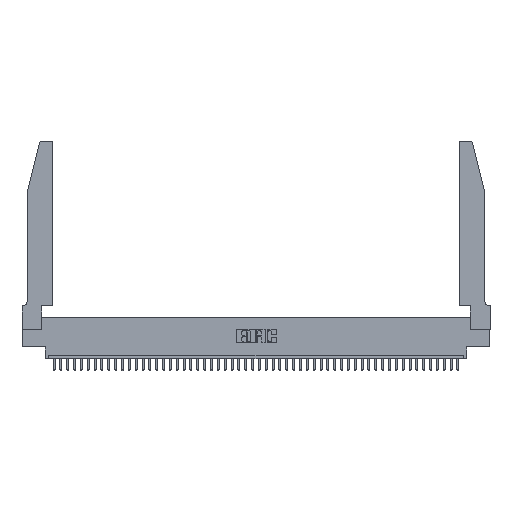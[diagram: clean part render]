
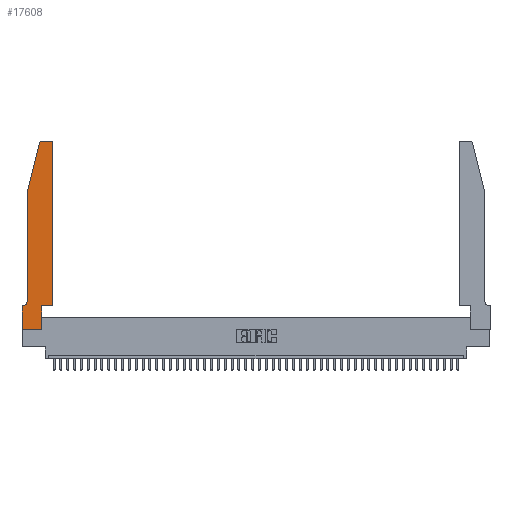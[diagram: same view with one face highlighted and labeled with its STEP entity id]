
A CAD part, top view. The second image highlights one B-rep face of the part: STEP entity #17608.
In plain terms, the highlighted planar face has unit normal (0, 0, 1).
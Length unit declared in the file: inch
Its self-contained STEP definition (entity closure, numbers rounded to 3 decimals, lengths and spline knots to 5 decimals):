
#796 = DIRECTION ( 'NONE',  ( -1., 0., 0. ) ) ;
#1854 = EDGE_CURVE ( 'NONE', #3958, #19040, #8267, .T. ) ;
#1920 = VECTOR ( 'NONE', #33301, 39.37008 ) ;
#2193 = ORIENTED_EDGE ( 'NONE', *, *, #1854, .T. ) ;
#2580 = AXIS2_PLACEMENT_3D ( 'NONE', #46384, #35325, #5504 ) ;
#2740 = DIRECTION ( 'NONE',  ( 0., 0., 1. ) ) ;
#3282 = AXIS2_PLACEMENT_3D ( 'NONE', #24497, #2740, #17591 ) ;
#3696 = CARTESIAN_POINT ( 'NONE',  ( 0.4505, 2.72, 0.37 ) ) ;
#3958 = VERTEX_POINT ( 'NONE', #18969 ) ;
#4555 = CARTESIAN_POINT ( 'NONE',  ( 0.0755, 2., 0.37 ) ) ;
#5211 = DIRECTION ( 'NONE',  ( 1., 0., 0. ) ) ;
#5504 = DIRECTION ( 'NONE',  ( 1., 0., 0. ) ) ;
#5720 = EDGE_CURVE ( 'NONE', #38643, #15057, #46241, .T. ) ;
#5841 = CARTESIAN_POINT ( 'NONE',  ( 0.2865, 0., 0.37 ) ) ;
#7037 = AXIS2_PLACEMENT_3D ( 'NONE', #32216, #13870, #47004 ) ;
#7317 = VECTOR ( 'NONE', #17837, 39.37008 ) ;
#7429 = DIRECTION ( 'NONE',  ( 0., 1., 0. ) ) ;
#8213 = ORIENTED_EDGE ( 'NONE', *, *, #44456, .T. ) ;
#8267 = LINE ( 'NONE', #10928, #1920 ) ;
#8400 = LINE ( 'NONE', #16300, #43541 ) ;
#8529 = EDGE_LOOP ( 'NONE', ( #19194, #29245, #8213, #34890, #30174, #2193, #38964, #18700, #45059, #26383, #11440, #38813 ) ) ;
#8995 = EDGE_CURVE ( 'NONE', #22311, #42083, #8400, .T. ) ;
#9408 = CARTESIAN_POINT ( 'NONE',  ( 0.0755, 2., 0.37 ) ) ;
#9685 = VERTEX_POINT ( 'NONE', #5841 ) ;
#10928 = CARTESIAN_POINT ( 'NONE',  ( 0.0755, 0.35, 0.37 ) ) ;
#11302 = DIRECTION ( 'NONE',  ( -0.239, -0.971, 0. ) ) ;
#11440 = ORIENTED_EDGE ( 'NONE', *, *, #37654, .T. ) ;
#12511 = LINE ( 'NONE', #28490, #7317 ) ;
#12840 = VECTOR ( 'NONE', #42834, 39.37008 ) ;
#13010 = VERTEX_POINT ( 'NONE', #25895 ) ;
#13510 = DIRECTION ( 'NONE',  ( 1., 0., 0. ) ) ;
#13753 = EDGE_CURVE ( 'NONE', #42083, #31272, #33928, .T. ) ;
#13870 = DIRECTION ( 'NONE',  ( 0., 0., -1. ) ) ;
#13898 = VECTOR ( 'NONE', #28652, 39.37008 ) ;
#15057 = VERTEX_POINT ( 'NONE', #15859 ) ;
#15088 = DIRECTION ( 'NONE',  ( 1., 0., 0. ) ) ;
#15477 = LINE ( 'NONE', #24240, #20648 ) ;
#15517 = EDGE_CURVE ( 'NONE', #29585, #20359, #20282, .T. ) ;
#15859 = CARTESIAN_POINT ( 'NONE',  ( 0.4505, 0.35, 0.37 ) ) ;
#16300 = CARTESIAN_POINT ( 'NONE',  ( 0.2605, 2.75, 0.37 ) ) ;
#16350 = LINE ( 'NONE', #43923, #18137 ) ;
#17591 = DIRECTION ( 'NONE',  ( 1., 0., 0. ) ) ;
#17608 = ADVANCED_FACE ( 'NONE', ( #18392 ), #24908, .T. ) ;
#17837 = DIRECTION ( 'NONE',  ( 0., 1., 0. ) ) ;
#17948 = VECTOR ( 'NONE', #11302, 39.37008 ) ;
#18137 = VECTOR ( 'NONE', #7429, 39.37008 ) ;
#18363 = CARTESIAN_POINT ( 'NONE',  ( 0.0755, 0.42, 0.37 ) ) ;
#18392 = FACE_OUTER_BOUND ( 'NONE', #8529, .T. ) ;
#18700 = ORIENTED_EDGE ( 'NONE', *, *, #21808, .T. ) ;
#18969 = CARTESIAN_POINT ( 'NONE',  ( 0.0055, 0.35, 0.37 ) ) ;
#19040 = VERTEX_POINT ( 'NONE', #28020 ) ;
#19194 = ORIENTED_EDGE ( 'NONE', *, *, #8995, .T. ) ;
#20282 = LINE ( 'NONE', #9408, #12840 ) ;
#20359 = VERTEX_POINT ( 'NONE', #18363 ) ;
#20648 = VECTOR ( 'NONE', #5211, 39.37008 ) ;
#21347 = CARTESIAN_POINT ( 'NONE',  ( 0.2865, 0.35, 0.37 ) ) ;
#21808 = EDGE_CURVE ( 'NONE', #13010, #9685, #15477, .T. ) ;
#22004 = CARTESIAN_POINT ( 'NONE',  ( 0.4505, 0.35, 0.37 ) ) ;
#22311 = VERTEX_POINT ( 'NONE', #41716 ) ;
#23304 = VERTEX_POINT ( 'NONE', #3696 ) ;
#24240 = CARTESIAN_POINT ( 'NONE',  ( 0., 0., 0.37 ) ) ;
#24378 = CIRCLE ( 'NONE', #7037, 0.07 ) ;
#24497 = CARTESIAN_POINT ( 'NONE',  ( 0.4205, 2.72, 0.37 ) ) ;
#24908 = PLANE ( 'NONE',  #34875 ) ;
#25783 = CIRCLE ( 'NONE', #3282, 0.03 ) ;
#25895 = CARTESIAN_POINT ( 'NONE',  ( 0., 0., 0.37 ) ) ;
#25985 = LINE ( 'NONE', #29375, #17948 ) ;
#26383 = ORIENTED_EDGE ( 'NONE', *, *, #5720, .T. ) ;
#27004 = CARTESIAN_POINT ( 'NONE',  ( 0.25487, 2.72718, 0.37 ) ) ;
#28020 = CARTESIAN_POINT ( 'NONE',  ( 0., 0.35, 0.37 ) ) ;
#28490 = CARTESIAN_POINT ( 'NONE',  ( 0.2865, 0.35, 0.37 ) ) ;
#28652 = DIRECTION ( 'NONE',  ( 0., -1., 0. ) ) ;
#29245 = ORIENTED_EDGE ( 'NONE', *, *, #13753, .T. ) ;
#29375 = CARTESIAN_POINT ( 'NONE',  ( 0.0755, 2., 0.37 ) ) ;
#29585 = VERTEX_POINT ( 'NONE', #4555 ) ;
#30174 = ORIENTED_EDGE ( 'NONE', *, *, #46888, .T. ) ;
#31272 = VERTEX_POINT ( 'NONE', #27004 ) ;
#32216 = CARTESIAN_POINT ( 'NONE',  ( 0.0055, 0.42, 0.37 ) ) ;
#32307 = EDGE_CURVE ( 'NONE', #9685, #38643, #12511, .T. ) ;
#33301 = DIRECTION ( 'NONE',  ( -1., 0., 0. ) ) ;
#33928 = CIRCLE ( 'NONE', #2580, 0.03 ) ;
#34875 = AXIS2_PLACEMENT_3D ( 'NONE', #43052, #39363, #13510 ) ;
#34890 = ORIENTED_EDGE ( 'NONE', *, *, #15517, .T. ) ;
#35325 = DIRECTION ( 'NONE',  ( 0., 0., 1. ) ) ;
#37654 = EDGE_CURVE ( 'NONE', #15057, #23304, #16350, .T. ) ;
#38643 = VERTEX_POINT ( 'NONE', #21347 ) ;
#38656 = CARTESIAN_POINT ( 'NONE',  ( 0.284, 2.75, 0.37 ) ) ;
#38813 = ORIENTED_EDGE ( 'NONE', *, *, #46251, .T. ) ;
#38964 = ORIENTED_EDGE ( 'NONE', *, *, #40058, .T. ) ;
#39308 = VECTOR ( 'NONE', #15088, 39.37008 ) ;
#39363 = DIRECTION ( 'NONE',  ( 0., 0., 1. ) ) ;
#40058 = EDGE_CURVE ( 'NONE', #19040, #13010, #41975, .T. ) ;
#41716 = CARTESIAN_POINT ( 'NONE',  ( 0.4205, 2.75, 0.37 ) ) ;
#41975 = LINE ( 'NONE', #47256, #13898 ) ;
#42083 = VERTEX_POINT ( 'NONE', #38656 ) ;
#42834 = DIRECTION ( 'NONE',  ( 0., -1., 0. ) ) ;
#43052 = CARTESIAN_POINT ( 'NONE',  ( 0., 0.35, 0.37 ) ) ;
#43541 = VECTOR ( 'NONE', #796, 39.37008 ) ;
#43923 = CARTESIAN_POINT ( 'NONE',  ( 0.4505, 0.35, 0.37 ) ) ;
#44456 = EDGE_CURVE ( 'NONE', #31272, #29585, #25985, .T. ) ;
#45059 = ORIENTED_EDGE ( 'NONE', *, *, #32307, .T. ) ;
#46241 = LINE ( 'NONE', #22004, #39308 ) ;
#46251 = EDGE_CURVE ( 'NONE', #23304, #22311, #25783, .T. ) ;
#46384 = CARTESIAN_POINT ( 'NONE',  ( 0.284, 2.72, 0.37 ) ) ;
#46888 = EDGE_CURVE ( 'NONE', #20359, #3958, #24378, .T. ) ;
#47004 = DIRECTION ( 'NONE',  ( -1., 0., 0. ) ) ;
#47256 = CARTESIAN_POINT ( 'NONE',  ( 0., 0., 0.37 ) ) ;
